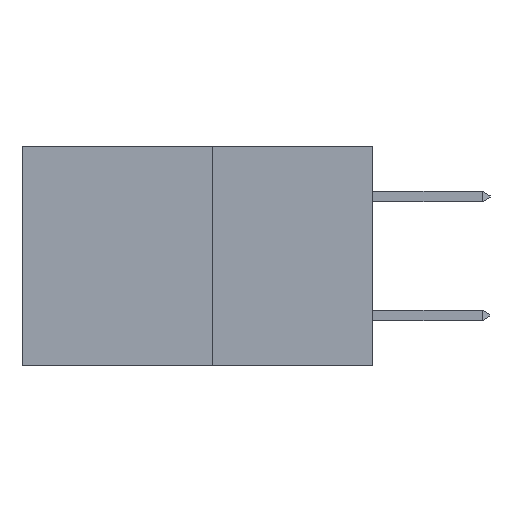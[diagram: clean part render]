
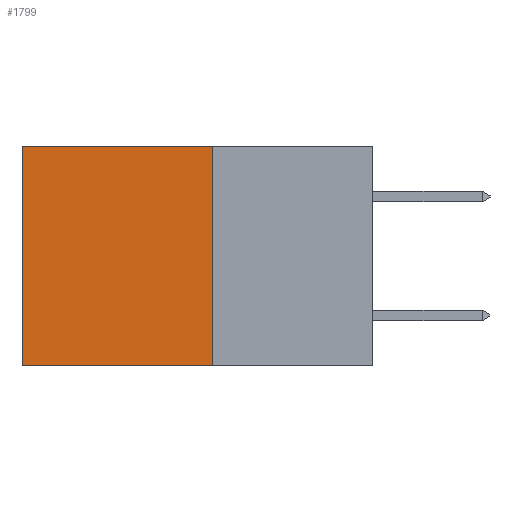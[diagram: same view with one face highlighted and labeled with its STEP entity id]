
A CAD part, left-side view. The second image highlights one B-rep face of the part: STEP entity #1799.
In plain terms, the highlighted planar face has unit normal (-1, 0, 0).
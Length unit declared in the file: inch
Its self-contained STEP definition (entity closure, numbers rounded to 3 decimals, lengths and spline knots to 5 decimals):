
#806 = VECTOR ( 'NONE', #10028, 39.37008 ) ;
#864 = VERTEX_POINT ( 'NONE', #7519 ) ;
#903 = DIRECTION ( 'NONE',  ( 0., 1., 0. ) ) ;
#962 = EDGE_CURVE ( 'NONE', #10397, #6772, #7781, .T. ) ;
#1130 = CARTESIAN_POINT ( 'NONE',  ( 0.277, 0.27, 0. ) ) ;
#1621 = EDGE_LOOP ( 'NONE', ( #3180, #13132, #7016, #10285 ) ) ;
#1799 = ADVANCED_FACE ( 'NONE', ( #11807 ), #9060, .F. ) ;
#2976 = CARTESIAN_POINT ( 'NONE',  ( 0.277, 0.27, 0. ) ) ;
#3027 = EDGE_CURVE ( 'NONE', #9584, #10397, #6197, .T. ) ;
#3180 = ORIENTED_EDGE ( 'NONE', *, *, #11660, .T. ) ;
#3295 = CARTESIAN_POINT ( 'NONE',  ( 0.277, 0.59, -0.37 ) ) ;
#4190 = AXIS2_PLACEMENT_3D ( 'NONE', #8692, #9507, #9484 ) ;
#4886 = CARTESIAN_POINT ( 'NONE',  ( 0.277, 0.27, -0.37 ) ) ;
#5787 = CARTESIAN_POINT ( 'NONE',  ( 0.277, 0.27, -0.37 ) ) ;
#6197 = LINE ( 'NONE', #10614, #15450 ) ;
#6772 = VERTEX_POINT ( 'NONE', #6985 ) ;
#6985 = CARTESIAN_POINT ( 'NONE',  ( 0.277, 0.59, -0.37 ) ) ;
#7016 = ORIENTED_EDGE ( 'NONE', *, *, #3027, .F. ) ;
#7155 = EDGE_CURVE ( 'NONE', #9584, #864, #15916, .T. ) ;
#7519 = CARTESIAN_POINT ( 'NONE',  ( 0.277, 0.59, 0. ) ) ;
#7781 = LINE ( 'NONE', #4886, #806 ) ;
#8692 = CARTESIAN_POINT ( 'NONE',  ( 0.277, 0.27, -0.37 ) ) ;
#9060 = PLANE ( 'NONE',  #4190 ) ;
#9484 = DIRECTION ( 'NONE',  ( 0., 0., -1. ) ) ;
#9507 = DIRECTION ( 'NONE',  ( 1., 0., 0. ) ) ;
#9551 = DIRECTION ( 'NONE',  ( 0., 0., -1. ) ) ;
#9584 = VERTEX_POINT ( 'NONE', #2976 ) ;
#10028 = DIRECTION ( 'NONE',  ( 0., 1., 0. ) ) ;
#10285 = ORIENTED_EDGE ( 'NONE', *, *, #7155, .T. ) ;
#10397 = VERTEX_POINT ( 'NONE', #5787 ) ;
#10406 = DIRECTION ( 'NONE',  ( 0., 0., -1. ) ) ;
#10614 = CARTESIAN_POINT ( 'NONE',  ( 0.277, 0.27, -0.37 ) ) ;
#11660 = EDGE_CURVE ( 'NONE', #864, #6772, #15784, .T. ) ;
#11807 = FACE_OUTER_BOUND ( 'NONE', #1621, .T. ) ;
#12684 = VECTOR ( 'NONE', #9551, 39.37008 ) ;
#12810 = VECTOR ( 'NONE', #903, 39.37008 ) ;
#13132 = ORIENTED_EDGE ( 'NONE', *, *, #962, .F. ) ;
#15450 = VECTOR ( 'NONE', #10406, 39.37008 ) ;
#15784 = LINE ( 'NONE', #3295, #12684 ) ;
#15916 = LINE ( 'NONE', #1130, #12810 ) ;
